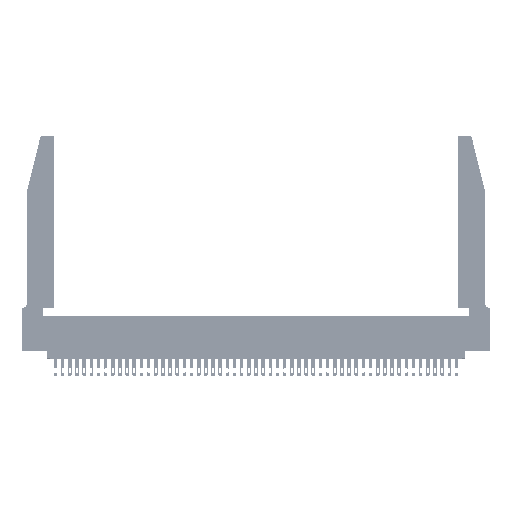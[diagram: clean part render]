
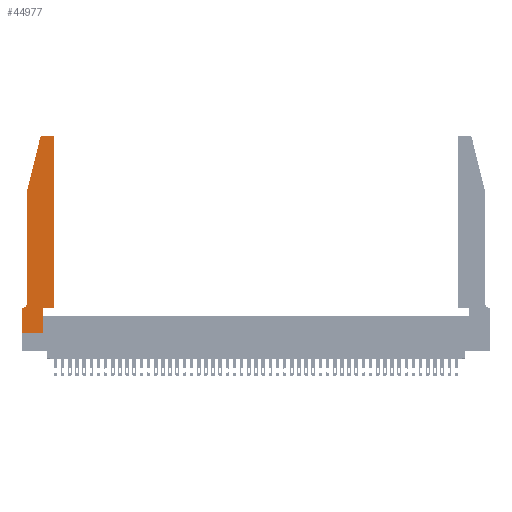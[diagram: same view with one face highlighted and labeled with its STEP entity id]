
A CAD part, top view. The second image highlights one B-rep face of the part: STEP entity #44977.
In plain terms, the highlighted planar face has unit normal (0, 0, 1).
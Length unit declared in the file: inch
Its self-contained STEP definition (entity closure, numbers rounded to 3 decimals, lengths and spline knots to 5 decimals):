
#105 = CARTESIAN_POINT ( 'NONE',  ( 0.0755, 0.35, 0.37 ) ) ;
#211 = VECTOR ( 'NONE', #8781, 39.37008 ) ;
#430 = LINE ( 'NONE', #34283, #20016 ) ;
#1541 = LINE ( 'NONE', #11966, #28079 ) ;
#2264 = EDGE_CURVE ( 'NONE', #45777, #10920, #1541, .T. ) ;
#2275 = DIRECTION ( 'NONE',  ( -1., 0., 0. ) ) ;
#3141 = VERTEX_POINT ( 'NONE', #11269 ) ;
#3237 = CIRCLE ( 'NONE', #28725, 0.03 ) ;
#3477 = VECTOR ( 'NONE', #28435, 39.37008 ) ;
#3536 = ORIENTED_EDGE ( 'NONE', *, *, #19359, .T. ) ;
#4086 = EDGE_CURVE ( 'NONE', #38930, #31806, #37031, .T. ) ;
#5215 = CARTESIAN_POINT ( 'NONE',  ( 0., 0., 0.37 ) ) ;
#5373 = CARTESIAN_POINT ( 'NONE',  ( 0.0055, 0.42, 0.37 ) ) ;
#6034 = CARTESIAN_POINT ( 'NONE',  ( 0.2865, 0.35, 0.37 ) ) ;
#6369 = VECTOR ( 'NONE', #7775, 39.37008 ) ;
#6557 = ORIENTED_EDGE ( 'NONE', *, *, #10489, .T. ) ;
#6890 = CARTESIAN_POINT ( 'NONE',  ( 0.0755, 0.42, 0.37 ) ) ;
#6954 = DIRECTION ( 'NONE',  ( 0., 1., 0. ) ) ;
#7487 = VECTOR ( 'NONE', #25334, 39.37008 ) ;
#7554 = CARTESIAN_POINT ( 'NONE',  ( 0.4505, 0.35, 0.37 ) ) ;
#7687 = DIRECTION ( 'NONE',  ( 0., 1., 0. ) ) ;
#7775 = DIRECTION ( 'NONE',  ( 0., -1., 0. ) ) ;
#8157 = ORIENTED_EDGE ( 'NONE', *, *, #37131, .T. ) ;
#8635 = DIRECTION ( 'NONE',  ( 1., 0., 0. ) ) ;
#8781 = DIRECTION ( 'NONE',  ( 1., 0., 0. ) ) ;
#8801 = CARTESIAN_POINT ( 'NONE',  ( 0., 0., 0.37 ) ) ;
#9010 = CARTESIAN_POINT ( 'NONE',  ( 0.2865, 0.35, 0.37 ) ) ;
#10314 = EDGE_CURVE ( 'NONE', #33601, #37893, #20429, .T. ) ;
#10489 = EDGE_CURVE ( 'NONE', #44076, #19412, #26902, .T. ) ;
#10920 = VERTEX_POINT ( 'NONE', #38691 ) ;
#11269 = CARTESIAN_POINT ( 'NONE',  ( 0., 0.35, 0.37 ) ) ;
#11544 = LINE ( 'NONE', #42047, #3477 ) ;
#11878 = DIRECTION ( 'NONE',  ( -1., 0., 0. ) ) ;
#11966 = CARTESIAN_POINT ( 'NONE',  ( 0.4505, 0.35, 0.37 ) ) ;
#12223 = EDGE_CURVE ( 'NONE', #10920, #33601, #3237, .T. ) ;
#12258 = DIRECTION ( 'NONE',  ( 0., 0., 1. ) ) ;
#12351 = DIRECTION ( 'NONE',  ( -0.239, -0.971, 0. ) ) ;
#13010 = CARTESIAN_POINT ( 'NONE',  ( 0.284, 2.72, 0.37 ) ) ;
#13036 = ORIENTED_EDGE ( 'NONE', *, *, #18117, .T. ) ;
#13812 = CARTESIAN_POINT ( 'NONE',  ( 0.2865, 0., 0.37 ) ) ;
#14340 = VECTOR ( 'NONE', #11878, 39.37008 ) ;
#16506 = VERTEX_POINT ( 'NONE', #6034 ) ;
#16742 = LINE ( 'NONE', #105, #7487 ) ;
#16786 = ORIENTED_EDGE ( 'NONE', *, *, #30538, .T. ) ;
#17511 = ORIENTED_EDGE ( 'NONE', *, *, #12223, .T. ) ;
#18117 = EDGE_CURVE ( 'NONE', #24031, #38930, #11544, .T. ) ;
#19087 = DIRECTION ( 'NONE',  ( 1., 0., 0. ) ) ;
#19330 = VERTEX_POINT ( 'NONE', #41175 ) ;
#19359 = EDGE_CURVE ( 'NONE', #19330, #24031, #430, .T. ) ;
#19412 = VERTEX_POINT ( 'NONE', #13812 ) ;
#20016 = VECTOR ( 'NONE', #12351, 39.37008 ) ;
#20429 = LINE ( 'NONE', #37338, #14340 ) ;
#20547 = ORIENTED_EDGE ( 'NONE', *, *, #4086, .T. ) ;
#22116 = ORIENTED_EDGE ( 'NONE', *, *, #41037, .T. ) ;
#23284 = CIRCLE ( 'NONE', #31541, 0.03 ) ;
#24031 = VERTEX_POINT ( 'NONE', #33223 ) ;
#24649 = CARTESIAN_POINT ( 'NONE',  ( 0.0055, 0.35, 0.37 ) ) ;
#25334 = DIRECTION ( 'NONE',  ( -1., 0., 0. ) ) ;
#25365 = EDGE_CURVE ( 'NONE', #16506, #45777, #47333, .T. ) ;
#26699 = ORIENTED_EDGE ( 'NONE', *, *, #10314, .T. ) ;
#26798 = EDGE_LOOP ( 'NONE', ( #26699, #22116, #3536, #13036, #20547, #31071, #8157, #6557, #16786, #43531, #27647, #17511 ) ) ;
#26902 = LINE ( 'NONE', #8801, #29791 ) ;
#27647 = ORIENTED_EDGE ( 'NONE', *, *, #2264, .T. ) ;
#28079 = VECTOR ( 'NONE', #6954, 39.37008 ) ;
#28435 = DIRECTION ( 'NONE',  ( 0., -1., 0. ) ) ;
#28725 = AXIS2_PLACEMENT_3D ( 'NONE', #41083, #12258, #19087 ) ;
#28803 = VECTOR ( 'NONE', #7687, 39.37008 ) ;
#29791 = VECTOR ( 'NONE', #8635, 39.37008 ) ;
#29792 = CARTESIAN_POINT ( 'NONE',  ( 0., 0., 0.37 ) ) ;
#30538 = EDGE_CURVE ( 'NONE', #19412, #16506, #38488, .T. ) ;
#31065 = AXIS2_PLACEMENT_3D ( 'NONE', #35491, #42870, #39114 ) ;
#31071 = ORIENTED_EDGE ( 'NONE', *, *, #43840, .T. ) ;
#31541 = AXIS2_PLACEMENT_3D ( 'NONE', #13010, #34773, #42484 ) ;
#31806 = VERTEX_POINT ( 'NONE', #24649 ) ;
#31807 = PLANE ( 'NONE',  #31065 ) ;
#32509 = AXIS2_PLACEMENT_3D ( 'NONE', #5373, #42433, #2275 ) ;
#33223 = CARTESIAN_POINT ( 'NONE',  ( 0.0755, 2., 0.37 ) ) ;
#33601 = VERTEX_POINT ( 'NONE', #34377 ) ;
#34283 = CARTESIAN_POINT ( 'NONE',  ( 0.0755, 2., 0.37 ) ) ;
#34377 = CARTESIAN_POINT ( 'NONE',  ( 0.4205, 2.75, 0.37 ) ) ;
#34387 = FACE_OUTER_BOUND ( 'NONE', #26798, .T. ) ;
#34773 = DIRECTION ( 'NONE',  ( 0., 0., 1. ) ) ;
#34874 = CARTESIAN_POINT ( 'NONE',  ( 0.284, 2.75, 0.37 ) ) ;
#35491 = CARTESIAN_POINT ( 'NONE',  ( 0., 0.35, 0.37 ) ) ;
#37031 = CIRCLE ( 'NONE', #32509, 0.07 ) ;
#37131 = EDGE_CURVE ( 'NONE', #3141, #44076, #37891, .T. ) ;
#37338 = CARTESIAN_POINT ( 'NONE',  ( 0.2605, 2.75, 0.37 ) ) ;
#37891 = LINE ( 'NONE', #29792, #6369 ) ;
#37893 = VERTEX_POINT ( 'NONE', #34874 ) ;
#38488 = LINE ( 'NONE', #9010, #28803 ) ;
#38691 = CARTESIAN_POINT ( 'NONE',  ( 0.4505, 2.72, 0.37 ) ) ;
#38930 = VERTEX_POINT ( 'NONE', #6890 ) ;
#39114 = DIRECTION ( 'NONE',  ( 1., 0., 0. ) ) ;
#41037 = EDGE_CURVE ( 'NONE', #37893, #19330, #23284, .T. ) ;
#41083 = CARTESIAN_POINT ( 'NONE',  ( 0.4205, 2.72, 0.37 ) ) ;
#41175 = CARTESIAN_POINT ( 'NONE',  ( 0.25487, 2.72718, 0.37 ) ) ;
#42047 = CARTESIAN_POINT ( 'NONE',  ( 0.0755, 2., 0.37 ) ) ;
#42433 = DIRECTION ( 'NONE',  ( 0., 0., -1. ) ) ;
#42484 = DIRECTION ( 'NONE',  ( 1., 0., 0. ) ) ;
#42870 = DIRECTION ( 'NONE',  ( 0., 0., 1. ) ) ;
#43531 = ORIENTED_EDGE ( 'NONE', *, *, #25365, .T. ) ;
#43840 = EDGE_CURVE ( 'NONE', #31806, #3141, #16742, .T. ) ;
#44076 = VERTEX_POINT ( 'NONE', #5215 ) ;
#44977 = ADVANCED_FACE ( 'NONE', ( #34387 ), #31807, .T. ) ;
#45707 = CARTESIAN_POINT ( 'NONE',  ( 0.4505, 0.35, 0.37 ) ) ;
#45777 = VERTEX_POINT ( 'NONE', #7554 ) ;
#47333 = LINE ( 'NONE', #45707, #211 ) ;
